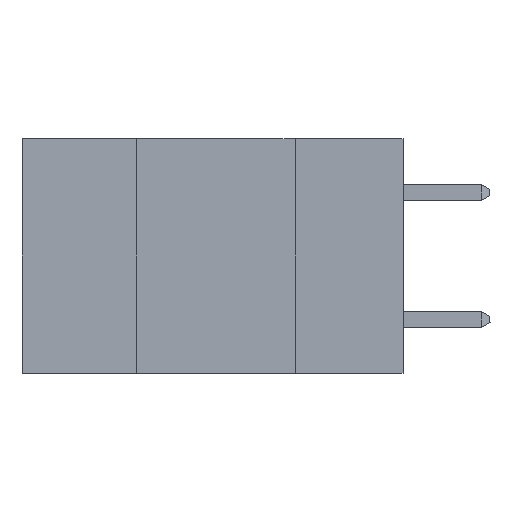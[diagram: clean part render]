
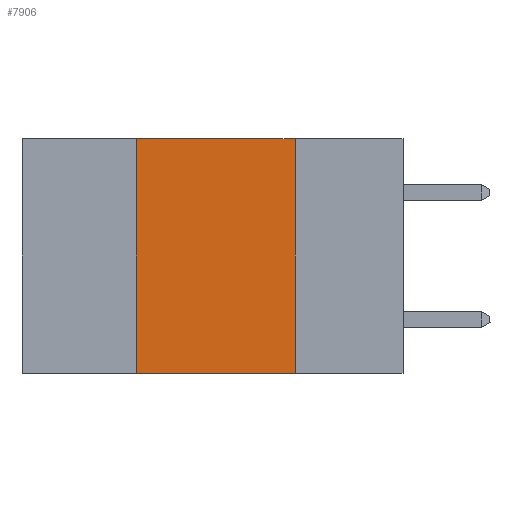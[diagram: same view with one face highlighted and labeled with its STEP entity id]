
A CAD part, left-side view. The second image highlights one B-rep face of the part: STEP entity #7906.
In plain terms, the highlighted planar face has unit normal (-1, 0, 0).
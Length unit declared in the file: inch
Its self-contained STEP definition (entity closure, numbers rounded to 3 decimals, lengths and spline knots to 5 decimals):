
#60 = ORIENTED_EDGE ( 'NONE', *, *, #14095, .F. ) ;
#407 = ORIENTED_EDGE ( 'NONE', *, *, #4499, .F. ) ;
#621 = CARTESIAN_POINT ( 'NONE',  ( 0., 0.42, -0.37 ) ) ;
#792 = CARTESIAN_POINT ( 'NONE',  ( 0., 0.6, 0. ) ) ;
#1483 = VERTEX_POINT ( 'NONE', #2509 ) ;
#2234 = EDGE_LOOP ( 'NONE', ( #60, #4088, #407, #3759 ) ) ;
#2509 = CARTESIAN_POINT ( 'NONE',  ( 0., 0.17, -0.37 ) ) ;
#2556 = DIRECTION ( 'NONE',  ( 0., 0., -1. ) ) ;
#3759 = ORIENTED_EDGE ( 'NONE', *, *, #13463, .T. ) ;
#3906 = PLANE ( 'NONE',  #9085 ) ;
#4088 = ORIENTED_EDGE ( 'NONE', *, *, #5452, .F. ) ;
#4215 = VECTOR ( 'NONE', #15064, 39.37008 ) ;
#4499 = EDGE_CURVE ( 'NONE', #14884, #13569, #18387, .T. ) ;
#4853 = DIRECTION ( 'NONE',  ( 0., -1., 0. ) ) ;
#5297 = CARTESIAN_POINT ( 'NONE',  ( 0., 0.6, 0. ) ) ;
#5452 = EDGE_CURVE ( 'NONE', #13569, #11331, #6738, .T. ) ;
#5671 = LINE ( 'NONE', #19469, #18173 ) ;
#6738 = LINE ( 'NONE', #5297, #19859 ) ;
#7545 = DIRECTION ( 'NONE',  ( 1., 0., 0. ) ) ;
#7906 = ADVANCED_FACE ( 'NONE', ( #19054 ), #3906, .F. ) ;
#8443 = CARTESIAN_POINT ( 'NONE',  ( 0., 0.42, 0. ) ) ;
#9085 = AXIS2_PLACEMENT_3D ( 'NONE', #792, #7545, #12400 ) ;
#10394 = VECTOR ( 'NONE', #4853, 39.37008 ) ;
#11331 = VERTEX_POINT ( 'NONE', #11845 ) ;
#11845 = CARTESIAN_POINT ( 'NONE',  ( 0., 0.17, 0. ) ) ;
#12400 = DIRECTION ( 'NONE',  ( 0., 0., -1. ) ) ;
#12437 = CARTESIAN_POINT ( 'NONE',  ( 0., 0.42, 0. ) ) ;
#13223 = CARTESIAN_POINT ( 'NONE',  ( 0., 0.6, -0.37 ) ) ;
#13463 = EDGE_CURVE ( 'NONE', #14884, #1483, #15212, .T. ) ;
#13569 = VERTEX_POINT ( 'NONE', #12437 ) ;
#14095 = EDGE_CURVE ( 'NONE', #11331, #1483, #5671, .T. ) ;
#14884 = VERTEX_POINT ( 'NONE', #621 ) ;
#15064 = DIRECTION ( 'NONE',  ( 0., 0., 1. ) ) ;
#15212 = LINE ( 'NONE', #13223, #10394 ) ;
#18173 = VECTOR ( 'NONE', #2556, 39.37008 ) ;
#18387 = LINE ( 'NONE', #8443, #4215 ) ;
#18553 = DIRECTION ( 'NONE',  ( 0., -1., 0. ) ) ;
#19054 = FACE_OUTER_BOUND ( 'NONE', #2234, .T. ) ;
#19469 = CARTESIAN_POINT ( 'NONE',  ( 0., 0.17, 0. ) ) ;
#19859 = VECTOR ( 'NONE', #18553, 39.37008 ) ;
